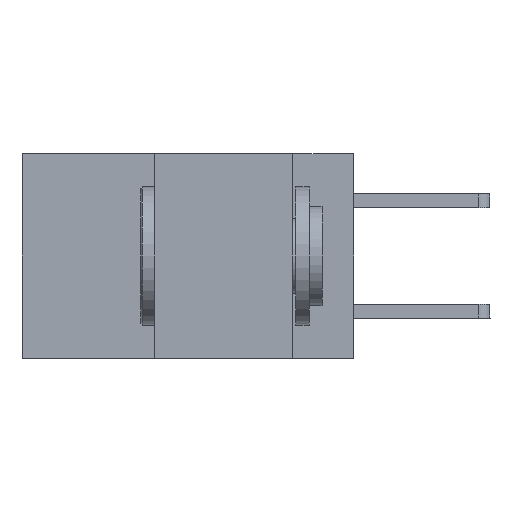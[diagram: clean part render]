
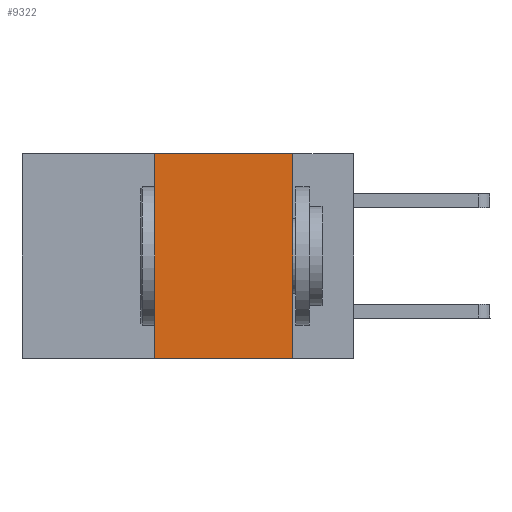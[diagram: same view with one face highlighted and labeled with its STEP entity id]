
A CAD part, left-side view. The second image highlights one B-rep face of the part: STEP entity #9322.
In plain terms, the highlighted planar face has unit normal (-1, 0, 0).
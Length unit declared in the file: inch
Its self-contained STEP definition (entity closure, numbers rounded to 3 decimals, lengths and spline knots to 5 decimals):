
#72 = EDGE_CURVE ( 'NONE', #2502, #1799, #12403, .T. ) ;
#932 = CARTESIAN_POINT ( 'NONE',  ( 0., 0.11, -0.37 ) ) ;
#934 = VECTOR ( 'NONE', #4794, 39.37008 ) ;
#1474 = LINE ( 'NONE', #7350, #934 ) ;
#1478 = DIRECTION ( 'NONE',  ( 0., 0., 1. ) ) ;
#1641 = DIRECTION ( 'NONE',  ( 0., -1., 0. ) ) ;
#1799 = VERTEX_POINT ( 'NONE', #2938 ) ;
#2502 = VERTEX_POINT ( 'NONE', #11814 ) ;
#2731 = CARTESIAN_POINT ( 'NONE',  ( 0., 0.36, 0. ) ) ;
#2813 = LINE ( 'NONE', #11308, #4744 ) ;
#2938 = CARTESIAN_POINT ( 'NONE',  ( 0., 0.36, 0. ) ) ;
#3653 = EDGE_CURVE ( 'NONE', #8360, #12016, #1474, .T. ) ;
#4369 = ORIENTED_EDGE ( 'NONE', *, *, #72, .F. ) ;
#4593 = EDGE_LOOP ( 'NONE', ( #7520, #13581, #4369, #9379 ) ) ;
#4744 = VECTOR ( 'NONE', #1641, 39.37008 ) ;
#4794 = DIRECTION ( 'NONE',  ( 0., 0., -1. ) ) ;
#5386 = CARTESIAN_POINT ( 'NONE',  ( 0., 0.11, 0. ) ) ;
#5754 = CARTESIAN_POINT ( 'NONE',  ( 0., 0.6, -0.37 ) ) ;
#7169 = CARTESIAN_POINT ( 'NONE',  ( 0., 0.6, 0. ) ) ;
#7204 = AXIS2_PLACEMENT_3D ( 'NONE', #7169, #11977, #8182 ) ;
#7350 = CARTESIAN_POINT ( 'NONE',  ( 0., 0.11, 0. ) ) ;
#7520 = ORIENTED_EDGE ( 'NONE', *, *, #3653, .F. ) ;
#8043 = FACE_OUTER_BOUND ( 'NONE', #4593, .T. ) ;
#8182 = DIRECTION ( 'NONE',  ( 0., 0., -1. ) ) ;
#8360 = VERTEX_POINT ( 'NONE', #5386 ) ;
#8405 = VECTOR ( 'NONE', #1478, 39.37008 ) ;
#9255 = VECTOR ( 'NONE', #13907, 39.37008 ) ;
#9322 = ADVANCED_FACE ( 'NONE', ( #8043 ), #13140, .F. ) ;
#9379 = ORIENTED_EDGE ( 'NONE', *, *, #10150, .T. ) ;
#10150 = EDGE_CURVE ( 'NONE', #2502, #12016, #13984, .T. ) ;
#11308 = CARTESIAN_POINT ( 'NONE',  ( 0., 0.6, 0. ) ) ;
#11814 = CARTESIAN_POINT ( 'NONE',  ( 0., 0.36, -0.37 ) ) ;
#11863 = EDGE_CURVE ( 'NONE', #1799, #8360, #2813, .T. ) ;
#11977 = DIRECTION ( 'NONE',  ( 1., 0., 0. ) ) ;
#12016 = VERTEX_POINT ( 'NONE', #932 ) ;
#12403 = LINE ( 'NONE', #2731, #8405 ) ;
#13140 = PLANE ( 'NONE',  #7204 ) ;
#13581 = ORIENTED_EDGE ( 'NONE', *, *, #11863, .F. ) ;
#13907 = DIRECTION ( 'NONE',  ( 0., -1., 0. ) ) ;
#13984 = LINE ( 'NONE', #5754, #9255 ) ;
